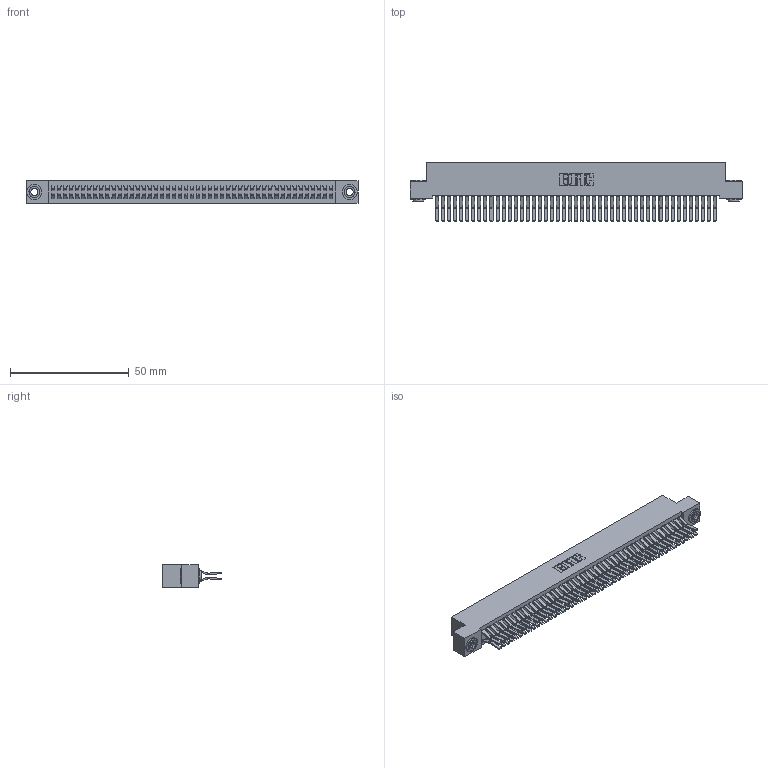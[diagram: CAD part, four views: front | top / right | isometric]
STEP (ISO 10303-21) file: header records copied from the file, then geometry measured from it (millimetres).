
FILE_DESCRIPTION (( 'STEP AP203' ), '1' );
FILE_NAME ('342-094-560-203.STEP', '2018-08-14T02:50:39', ( '' ), ( '' ), 'SwSTEP 2.0', 'SolidWorks 2016', '' );
FILE_SCHEMA (( 'CONFIG_CONTROL_DESIGN' ));
Length unit declared in the file: inch
Products named in the file (4): 342 Part_.156 TH; 345-292-001_560 Tail; 342-250-002_345-250-002-102; 342-094-560-203
Assembly tree (97 placements, depth 2):
  342-094-560-203
    342 Part_.156 TH
    345-292-001_560 Tail  x94
    342-250-002_345-250-002-102  x2
Bounding box: 139.7 x 24.78 x 9.4 mm (x, y, z)
Volume: 13215.7 mm3; surface area: 23328.9 mm2
Topology: 97 solids, 97 shells, 5224 faces, 15509 edges, 10210 vertices
Faces by surface type: plane 3460, cylinder 1756, cone 8
Entity records: 30196 total; most frequent: CARTESIAN_POINT 4973, ORIENTED_EDGE 4902, DIRECTION 4277, EDGE_CURVE 2451, LINE 2295, VECTOR 2295, VERTEX_POINT 1630, AXIS2_PLACEMENT_3D 991
